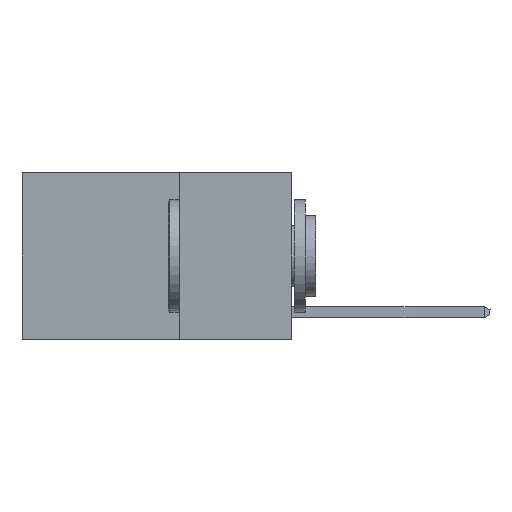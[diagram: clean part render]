
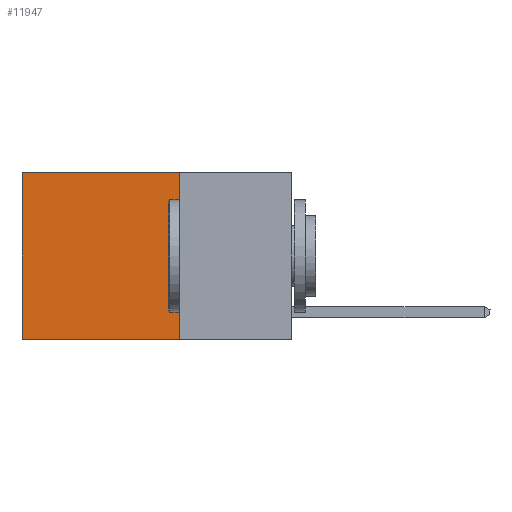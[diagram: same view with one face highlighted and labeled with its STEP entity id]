
A CAD part, left-side view. The second image highlights one B-rep face of the part: STEP entity #11947.
In plain terms, the highlighted planar face has unit normal (-1, 0, 0).
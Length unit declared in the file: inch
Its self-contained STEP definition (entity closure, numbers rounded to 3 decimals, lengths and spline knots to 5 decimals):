
#188 = VERTEX_POINT ( 'NONE', #17044 ) ;
#428 = EDGE_CURVE ( 'NONE', #4679, #188, #3887, .T. ) ;
#1403 = LINE ( 'NONE', #2155, #21104 ) ;
#1435 = FACE_OUTER_BOUND ( 'NONE', #6992, .T. ) ;
#1695 = AXIS2_PLACEMENT_3D ( 'NONE', #17239, #22437, #11957 ) ;
#2062 = VERTEX_POINT ( 'NONE', #5035 ) ;
#2155 = CARTESIAN_POINT ( 'NONE',  ( 0.2625, 0.25, 0. ) ) ;
#2678 = CARTESIAN_POINT ( 'NONE',  ( 0.2625, 0.25, -0.37 ) ) ;
#3562 = CARTESIAN_POINT ( 'NONE',  ( 0.2625, 0.25, 0. ) ) ;
#3887 = LINE ( 'NONE', #10992, #22168 ) ;
#4679 = VERTEX_POINT ( 'NONE', #8848 ) ;
#5035 = CARTESIAN_POINT ( 'NONE',  ( 0.2625, 0.25, -0.37 ) ) ;
#6992 = EDGE_LOOP ( 'NONE', ( #17715, #22099, #23286, #8084 ) ) ;
#7037 = CARTESIAN_POINT ( 'NONE',  ( 0.2625, 0.25, 0. ) ) ;
#7237 = EDGE_CURVE ( 'NONE', #17535, #4679, #1403, .T. ) ;
#8084 = ORIENTED_EDGE ( 'NONE', *, *, #7237, .T. ) ;
#8531 = EDGE_CURVE ( 'NONE', #2062, #188, #8779, .T. ) ;
#8779 = LINE ( 'NONE', #2678, #22368 ) ;
#8848 = CARTESIAN_POINT ( 'NONE',  ( 0.2625, 0.6, 0. ) ) ;
#9035 = DIRECTION ( 'NONE',  ( 0., 0., -1. ) ) ;
#9247 = LINE ( 'NONE', #7037, #18209 ) ;
#10124 = PLANE ( 'NONE',  #1695 ) ;
#10789 = DIRECTION ( 'NONE',  ( 0., 0., -1. ) ) ;
#10992 = CARTESIAN_POINT ( 'NONE',  ( 0.2625, 0.6, 0. ) ) ;
#11039 = EDGE_CURVE ( 'NONE', #17535, #2062, #9247, .T. ) ;
#11947 = ADVANCED_FACE ( 'NONE', ( #1435 ), #10124, .F. ) ;
#11957 = DIRECTION ( 'NONE',  ( 0., 0., -1. ) ) ;
#14116 = DIRECTION ( 'NONE',  ( 0., 1., 0. ) ) ;
#15406 = DIRECTION ( 'NONE',  ( 0., 1., 0. ) ) ;
#17044 = CARTESIAN_POINT ( 'NONE',  ( 0.2625, 0.6, -0.37 ) ) ;
#17239 = CARTESIAN_POINT ( 'NONE',  ( 0.2625, 0.25, 0. ) ) ;
#17535 = VERTEX_POINT ( 'NONE', #3562 ) ;
#17715 = ORIENTED_EDGE ( 'NONE', *, *, #428, .T. ) ;
#18209 = VECTOR ( 'NONE', #9035, 39.37008 ) ;
#21104 = VECTOR ( 'NONE', #15406, 39.37008 ) ;
#22099 = ORIENTED_EDGE ( 'NONE', *, *, #8531, .F. ) ;
#22168 = VECTOR ( 'NONE', #10789, 39.37008 ) ;
#22368 = VECTOR ( 'NONE', #14116, 39.37008 ) ;
#22437 = DIRECTION ( 'NONE',  ( 1., 0., 0. ) ) ;
#23286 = ORIENTED_EDGE ( 'NONE', *, *, #11039, .F. ) ;
